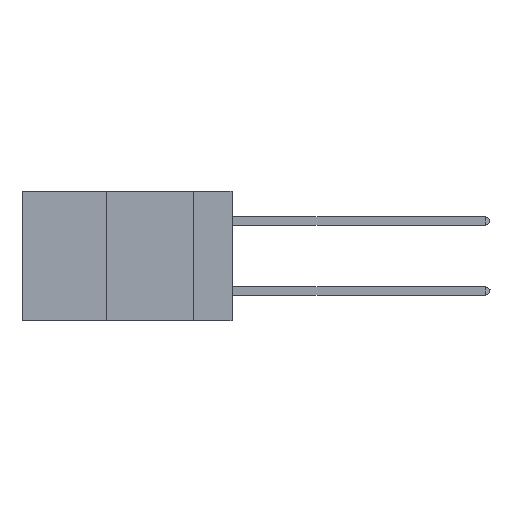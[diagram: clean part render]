
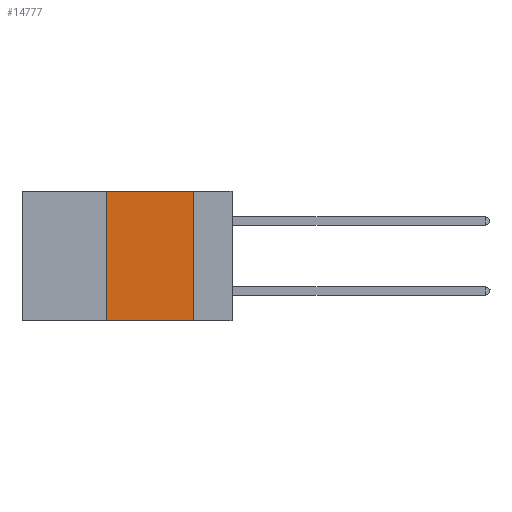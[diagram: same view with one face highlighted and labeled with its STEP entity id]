
A CAD part, left-side view. The second image highlights one B-rep face of the part: STEP entity #14777.
In plain terms, the highlighted planar face has unit normal (-1, 0, 0).
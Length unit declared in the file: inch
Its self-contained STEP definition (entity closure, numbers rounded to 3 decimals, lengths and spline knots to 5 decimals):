
#307 = EDGE_CURVE ( 'NONE', #4643, #1204, #4318, .T. ) ;
#833 = VECTOR ( 'NONE', #21436, 39.37008 ) ;
#876 = LINE ( 'NONE', #15316, #11013 ) ;
#1204 = VERTEX_POINT ( 'NONE', #1649 ) ;
#1649 = CARTESIAN_POINT ( 'NONE',  ( 0., 0.11, -0.37 ) ) ;
#2438 = CARTESIAN_POINT ( 'NONE',  ( 0., 0.6, 0. ) ) ;
#2664 = CARTESIAN_POINT ( 'NONE',  ( 0., 0.36, 0. ) ) ;
#3034 = VECTOR ( 'NONE', #4390, 39.37008 ) ;
#3926 = ORIENTED_EDGE ( 'NONE', *, *, #307, .T. ) ;
#4318 = LINE ( 'NONE', #13054, #833 ) ;
#4390 = DIRECTION ( 'NONE',  ( 0., -1., 0. ) ) ;
#4643 = VERTEX_POINT ( 'NONE', #19487 ) ;
#5043 = CARTESIAN_POINT ( 'NONE',  ( 0., 0.11, 0. ) ) ;
#5461 = EDGE_CURVE ( 'NONE', #15526, #13495, #10239, .T. ) ;
#7469 = ORIENTED_EDGE ( 'NONE', *, *, #5461, .F. ) ;
#7915 = FACE_OUTER_BOUND ( 'NONE', #10737, .T. ) ;
#9367 = CARTESIAN_POINT ( 'NONE',  ( 0., 0.6, 0. ) ) ;
#10239 = LINE ( 'NONE', #9367, #3034 ) ;
#10737 = EDGE_LOOP ( 'NONE', ( #16138, #7469, #18570, #3926 ) ) ;
#11013 = VECTOR ( 'NONE', #18502, 39.37008 ) ;
#11658 = DIRECTION ( 'NONE',  ( 0., 0., -1. ) ) ;
#12693 = DIRECTION ( 'NONE',  ( 0., 0., -1. ) ) ;
#13054 = CARTESIAN_POINT ( 'NONE',  ( 0., 0.6, -0.37 ) ) ;
#13495 = VERTEX_POINT ( 'NONE', #21000 ) ;
#14777 = ADVANCED_FACE ( 'NONE', ( #7915 ), #21460, .F. ) ;
#15095 = DIRECTION ( 'NONE',  ( 1., 0., 0. ) ) ;
#15316 = CARTESIAN_POINT ( 'NONE',  ( 0., 0.36, 0. ) ) ;
#15526 = VERTEX_POINT ( 'NONE', #2664 ) ;
#16138 = ORIENTED_EDGE ( 'NONE', *, *, #18511, .F. ) ;
#17066 = VECTOR ( 'NONE', #11658, 39.37008 ) ;
#17127 = EDGE_CURVE ( 'NONE', #4643, #15526, #876, .T. ) ;
#18083 = AXIS2_PLACEMENT_3D ( 'NONE', #2438, #15095, #12693 ) ;
#18502 = DIRECTION ( 'NONE',  ( 0., 0., 1. ) ) ;
#18511 = EDGE_CURVE ( 'NONE', #13495, #1204, #21605, .T. ) ;
#18570 = ORIENTED_EDGE ( 'NONE', *, *, #17127, .F. ) ;
#19487 = CARTESIAN_POINT ( 'NONE',  ( 0., 0.36, -0.37 ) ) ;
#21000 = CARTESIAN_POINT ( 'NONE',  ( 0., 0.11, 0. ) ) ;
#21436 = DIRECTION ( 'NONE',  ( 0., -1., 0. ) ) ;
#21460 = PLANE ( 'NONE',  #18083 ) ;
#21605 = LINE ( 'NONE', #5043, #17066 ) ;
